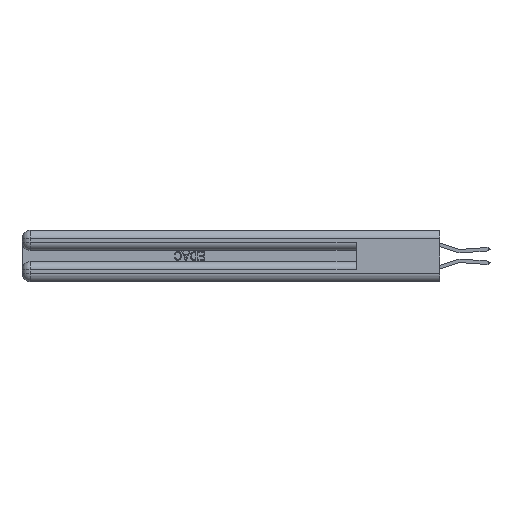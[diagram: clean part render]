
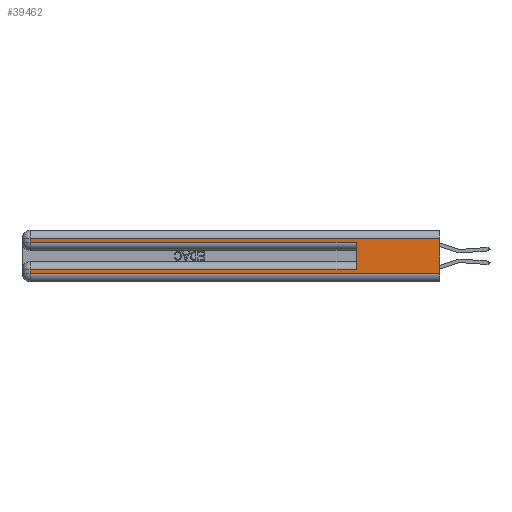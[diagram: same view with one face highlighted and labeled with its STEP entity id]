
A CAD part, left-side view. The second image highlights one B-rep face of the part: STEP entity #39462.
In plain terms, the highlighted planar face has unit normal (-1, 0, 0).
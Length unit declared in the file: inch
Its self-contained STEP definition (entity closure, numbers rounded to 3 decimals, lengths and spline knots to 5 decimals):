
#648 = VECTOR ( 'NONE', #15209, 39.37008 ) ;
#2213 = CARTESIAN_POINT ( 'NONE',  ( 0., 0., 0.06 ) ) ;
#2757 = DIRECTION ( 'NONE',  ( 0., 0., 1. ) ) ;
#2863 = DIRECTION ( 'NONE',  ( 0., 1., 0. ) ) ;
#3060 = LINE ( 'NONE', #2213, #37608 ) ;
#3195 = ORIENTED_EDGE ( 'NONE', *, *, #31838, .T. ) ;
#3972 = PLANE ( 'NONE',  #30613 ) ;
#4170 = CARTESIAN_POINT ( 'NONE',  ( 0., 2.94, 0.37 ) ) ;
#5823 = LINE ( 'NONE', #7903, #36856 ) ;
#6708 = EDGE_CURVE ( 'NONE', #22243, #39316, #5823, .T. ) ;
#7377 = CARTESIAN_POINT ( 'NONE',  ( 0., 2.94, 0.06 ) ) ;
#7584 = EDGE_CURVE ( 'NONE', #40252, #19124, #26628, .T. ) ;
#7903 = CARTESIAN_POINT ( 'NONE',  ( 0., 0., 0.285 ) ) ;
#7915 = VECTOR ( 'NONE', #10703, 39.37008 ) ;
#8003 = EDGE_CURVE ( 'NONE', #19816, #39316, #41455, .T. ) ;
#9349 = LINE ( 'NONE', #4170, #648 ) ;
#10008 = EDGE_CURVE ( 'NONE', #26570, #22243, #9349, .T. ) ;
#10703 = DIRECTION ( 'NONE',  ( 0., 1., 0. ) ) ;
#11164 = ORIENTED_EDGE ( 'NONE', *, *, #37799, .T. ) ;
#12530 = VERTEX_POINT ( 'NONE', #7377 ) ;
#13615 = CARTESIAN_POINT ( 'NONE',  ( 0., 0., 0.37 ) ) ;
#13732 = DIRECTION ( 'NONE',  ( 0., 0., -1. ) ) ;
#13890 = VECTOR ( 'NONE', #15718, 39.37008 ) ;
#14728 = ORIENTED_EDGE ( 'NONE', *, *, #10008, .T. ) ;
#15209 = DIRECTION ( 'NONE',  ( 0., 0., -1. ) ) ;
#15380 = EDGE_CURVE ( 'NONE', #40252, #26570, #38995, .T. ) ;
#15718 = DIRECTION ( 'NONE',  ( 0., 0., -1. ) ) ;
#16788 = EDGE_CURVE ( 'NONE', #39819, #12530, #30266, .T. ) ;
#17511 = CARTESIAN_POINT ( 'NONE',  ( 0., 0., 0.31 ) ) ;
#19124 = VERTEX_POINT ( 'NONE', #34512 ) ;
#19816 = VERTEX_POINT ( 'NONE', #32889 ) ;
#21407 = ORIENTED_EDGE ( 'NONE', *, *, #15380, .T. ) ;
#22243 = VERTEX_POINT ( 'NONE', #40661 ) ;
#24044 = ORIENTED_EDGE ( 'NONE', *, *, #8003, .F. ) ;
#24519 = FACE_OUTER_BOUND ( 'NONE', #41789, .T. ) ;
#26570 = VERTEX_POINT ( 'NONE', #27727 ) ;
#26628 = LINE ( 'NONE', #40823, #13890 ) ;
#26672 = VECTOR ( 'NONE', #41824, 39.37008 ) ;
#27727 = CARTESIAN_POINT ( 'NONE',  ( 0., 2.94, 0.31 ) ) ;
#28094 = ORIENTED_EDGE ( 'NONE', *, *, #7584, .F. ) ;
#28481 = DIRECTION ( 'NONE',  ( 0., -1., 0. ) ) ;
#28690 = CARTESIAN_POINT ( 'NONE',  ( 0., 2.94, 0.085 ) ) ;
#29164 = CARTESIAN_POINT ( 'NONE',  ( 0., 0.6, 0.145 ) ) ;
#30046 = CARTESIAN_POINT ( 'NONE',  ( 0., 0., 0.31 ) ) ;
#30266 = LINE ( 'NONE', #34833, #26672 ) ;
#30613 = AXIS2_PLACEMENT_3D ( 'NONE', #13615, #32845, #13732 ) ;
#30641 = DIRECTION ( 'NONE',  ( 0., -1., 0. ) ) ;
#31838 = EDGE_CURVE ( 'NONE', #12530, #19124, #3060, .T. ) ;
#32120 = CARTESIAN_POINT ( 'NONE',  ( 0., 0., 0.085 ) ) ;
#32168 = ORIENTED_EDGE ( 'NONE', *, *, #6708, .T. ) ;
#32236 = VECTOR ( 'NONE', #2757, 39.37008 ) ;
#32845 = DIRECTION ( 'NONE',  ( 1., 0., 0. ) ) ;
#32889 = CARTESIAN_POINT ( 'NONE',  ( 0., 0.6, 0.085 ) ) ;
#33458 = VECTOR ( 'NONE', #2863, 39.37008 ) ;
#34164 = ORIENTED_EDGE ( 'NONE', *, *, #16788, .T. ) ;
#34512 = CARTESIAN_POINT ( 'NONE',  ( 0., 0., 0.06 ) ) ;
#34833 = CARTESIAN_POINT ( 'NONE',  ( 0., 2.94, 0.37 ) ) ;
#35439 = CARTESIAN_POINT ( 'NONE',  ( 0., 0.6, 0.285 ) ) ;
#36856 = VECTOR ( 'NONE', #30641, 39.37008 ) ;
#37608 = VECTOR ( 'NONE', #28481, 39.37008 ) ;
#37799 = EDGE_CURVE ( 'NONE', #19816, #39819, #40619, .T. ) ;
#38995 = LINE ( 'NONE', #30046, #7915 ) ;
#39316 = VERTEX_POINT ( 'NONE', #35439 ) ;
#39462 = ADVANCED_FACE ( 'NONE', ( #24519 ), #3972, .F. ) ;
#39819 = VERTEX_POINT ( 'NONE', #28690 ) ;
#40252 = VERTEX_POINT ( 'NONE', #17511 ) ;
#40619 = LINE ( 'NONE', #32120, #33458 ) ;
#40661 = CARTESIAN_POINT ( 'NONE',  ( 0., 2.94, 0.285 ) ) ;
#40823 = CARTESIAN_POINT ( 'NONE',  ( 0., 0., 0.37 ) ) ;
#41455 = LINE ( 'NONE', #29164, #32236 ) ;
#41789 = EDGE_LOOP ( 'NONE', ( #28094, #21407, #14728, #32168, #24044, #11164, #34164, #3195 ) ) ;
#41824 = DIRECTION ( 'NONE',  ( 0., 0., -1. ) ) ;
